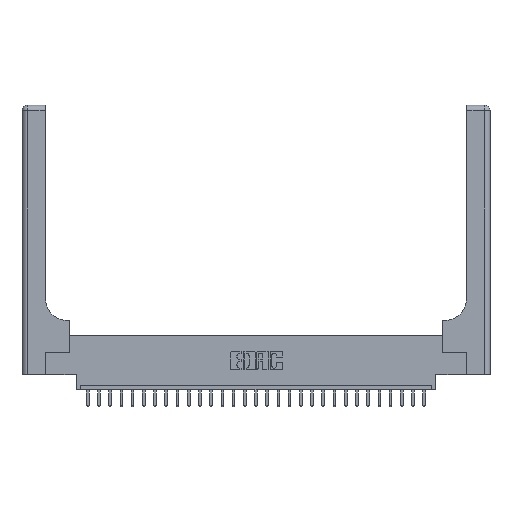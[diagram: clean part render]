
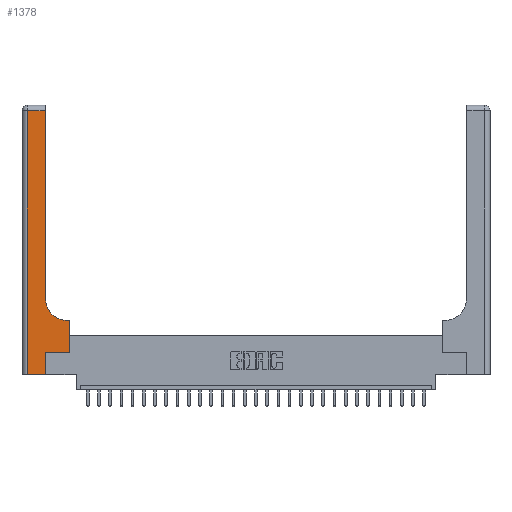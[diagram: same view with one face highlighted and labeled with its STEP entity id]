
A CAD part, top view. The second image highlights one B-rep face of the part: STEP entity #1378.
In plain terms, the highlighted planar face has unit normal (0, 0, 1).
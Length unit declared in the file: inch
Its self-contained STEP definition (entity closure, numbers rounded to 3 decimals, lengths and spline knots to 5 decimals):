
#439 = DIRECTION ( 'NONE',  ( 0., -1., 0. ) ) ;
#1042 = CARTESIAN_POINT ( 'NONE',  ( 0.528, 0.25, 0.37 ) ) ;
#1378 = ADVANCED_FACE ( 'NONE', ( #7608 ), #21577, .F. ) ;
#1448 = EDGE_LOOP ( 'NONE', ( #8449, #17244, #14795, #13233, #22010, #15923, #24843, #17185, #17622 ) ) ;
#2516 = EDGE_CURVE ( 'NONE', #13386, #11999, #22420, .T. ) ;
#2590 = DIRECTION ( 'NONE',  ( 0., 0., -1. ) ) ;
#2871 = DIRECTION ( 'NONE',  ( 1., 0., 0. ) ) ;
#2874 = VERTEX_POINT ( 'NONE', #15776 ) ;
#3213 = DIRECTION ( 'NONE',  ( -1., 0., 0. ) ) ;
#3817 = CARTESIAN_POINT ( 'NONE',  ( 0.06, 0., 0.37 ) ) ;
#3854 = VECTOR ( 'NONE', #23602, 39.37008 ) ;
#3879 = CARTESIAN_POINT ( 'NONE',  ( 0.265, 0., 0.37 ) ) ;
#4439 = CARTESIAN_POINT ( 'NONE',  ( 0.528, 0.25, 0.37 ) ) ;
#4842 = LINE ( 'NONE', #23786, #3854 ) ;
#5367 = LINE ( 'NONE', #17953, #6011 ) ;
#5626 = EDGE_CURVE ( 'NONE', #26090, #2874, #23275, .T. ) ;
#5753 = DIRECTION ( 'NONE',  ( 0., 1., 0. ) ) ;
#5790 = DIRECTION ( 'NONE',  ( -1., 0., 0. ) ) ;
#5980 = CIRCLE ( 'NONE', #7680, 0.25 ) ;
#6011 = VECTOR ( 'NONE', #5790, 39.37008 ) ;
#6057 = EDGE_CURVE ( 'NONE', #22984, #20961, #5980, .T. ) ;
#6498 = EDGE_CURVE ( 'NONE', #23726, #7362, #21747, .T. ) ;
#6804 = VERTEX_POINT ( 'NONE', #18829 ) ;
#7362 = VERTEX_POINT ( 'NONE', #3817 ) ;
#7608 = FACE_OUTER_BOUND ( 'NONE', #1448, .T. ) ;
#7618 = CARTESIAN_POINT ( 'NONE',  ( 0., 0., 0.37 ) ) ;
#7680 = AXIS2_PLACEMENT_3D ( 'NONE', #23361, #2590, #12657 ) ;
#8449 = ORIENTED_EDGE ( 'NONE', *, *, #19237, .T. ) ;
#9198 = EDGE_CURVE ( 'NONE', #11999, #26090, #23231, .T. ) ;
#9774 = CARTESIAN_POINT ( 'NONE',  ( 0.26, 3., 0.37 ) ) ;
#10955 = VECTOR ( 'NONE', #13805, 39.37008 ) ;
#11042 = CARTESIAN_POINT ( 'NONE',  ( 0.26, 0.85, 0.37 ) ) ;
#11482 = DIRECTION ( 'NONE',  ( 0., 0., -1. ) ) ;
#11645 = AXIS2_PLACEMENT_3D ( 'NONE', #17257, #11482, #3213 ) ;
#11999 = VERTEX_POINT ( 'NONE', #23550 ) ;
#12657 = DIRECTION ( 'NONE',  ( 1., 0., 0. ) ) ;
#12849 = CARTESIAN_POINT ( 'NONE',  ( 0.265, 0.25, 0.37 ) ) ;
#12949 = LINE ( 'NONE', #9774, #13245 ) ;
#13233 = ORIENTED_EDGE ( 'NONE', *, *, #15467, .T. ) ;
#13245 = VECTOR ( 'NONE', #23923, 39.37008 ) ;
#13386 = VERTEX_POINT ( 'NONE', #3879 ) ;
#13805 = DIRECTION ( 'NONE',  ( 1., 0., 0. ) ) ;
#14795 = ORIENTED_EDGE ( 'NONE', *, *, #6498, .T. ) ;
#15467 = EDGE_CURVE ( 'NONE', #7362, #13386, #16030, .T. ) ;
#15776 = CARTESIAN_POINT ( 'NONE',  ( 0.528, 0.6, 0.37 ) ) ;
#15923 = ORIENTED_EDGE ( 'NONE', *, *, #9198, .T. ) ;
#16030 = LINE ( 'NONE', #7618, #10955 ) ;
#16608 = DIRECTION ( 'NONE',  ( 0., 1., 0. ) ) ;
#17185 = ORIENTED_EDGE ( 'NONE', *, *, #25063, .T. ) ;
#17244 = ORIENTED_EDGE ( 'NONE', *, *, #23685, .T. ) ;
#17257 = CARTESIAN_POINT ( 'NONE',  ( 0., 3., 0.37 ) ) ;
#17622 = ORIENTED_EDGE ( 'NONE', *, *, #6057, .T. ) ;
#17839 = VECTOR ( 'NONE', #2871, 39.37008 ) ;
#17953 = CARTESIAN_POINT ( 'NONE',  ( 0.26, 0.6, 0.37 ) ) ;
#18829 = CARTESIAN_POINT ( 'NONE',  ( 0.26, 2.94, 0.37 ) ) ;
#19237 = EDGE_CURVE ( 'NONE', #20961, #6804, #12949, .T. ) ;
#19827 = VECTOR ( 'NONE', #439, 39.37008 ) ;
#20961 = VERTEX_POINT ( 'NONE', #11042 ) ;
#21577 = PLANE ( 'NONE',  #11645 ) ;
#21673 = CARTESIAN_POINT ( 'NONE',  ( 0.06, 2.94, 0.37 ) ) ;
#21747 = LINE ( 'NONE', #22807, #19827 ) ;
#21908 = CARTESIAN_POINT ( 'NONE',  ( 0.265, 0., 0.37 ) ) ;
#21976 = VECTOR ( 'NONE', #16608, 39.37008 ) ;
#22010 = ORIENTED_EDGE ( 'NONE', *, *, #2516, .T. ) ;
#22420 = LINE ( 'NONE', #21908, #23069 ) ;
#22807 = CARTESIAN_POINT ( 'NONE',  ( 0.06, 3., 0.37 ) ) ;
#22984 = VERTEX_POINT ( 'NONE', #25490 ) ;
#23069 = VECTOR ( 'NONE', #5753, 39.37008 ) ;
#23231 = LINE ( 'NONE', #12849, #17839 ) ;
#23275 = LINE ( 'NONE', #4439, #21976 ) ;
#23361 = CARTESIAN_POINT ( 'NONE',  ( 0.51, 0.85, 0.37 ) ) ;
#23550 = CARTESIAN_POINT ( 'NONE',  ( 0.265, 0.25, 0.37 ) ) ;
#23602 = DIRECTION ( 'NONE',  ( -1., 0., 0. ) ) ;
#23685 = EDGE_CURVE ( 'NONE', #6804, #23726, #4842, .T. ) ;
#23726 = VERTEX_POINT ( 'NONE', #21673 ) ;
#23786 = CARTESIAN_POINT ( 'NONE',  ( 0., 2.94, 0.37 ) ) ;
#23923 = DIRECTION ( 'NONE',  ( 0., 1., 0. ) ) ;
#24843 = ORIENTED_EDGE ( 'NONE', *, *, #5626, .T. ) ;
#25063 = EDGE_CURVE ( 'NONE', #2874, #22984, #5367, .T. ) ;
#25490 = CARTESIAN_POINT ( 'NONE',  ( 0.51, 0.6, 0.37 ) ) ;
#26090 = VERTEX_POINT ( 'NONE', #1042 ) ;
